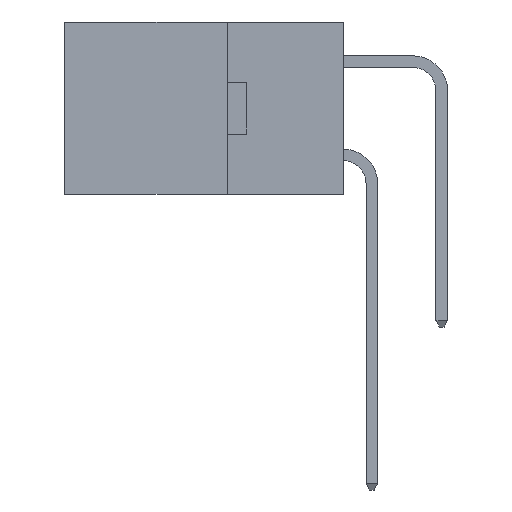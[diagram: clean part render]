
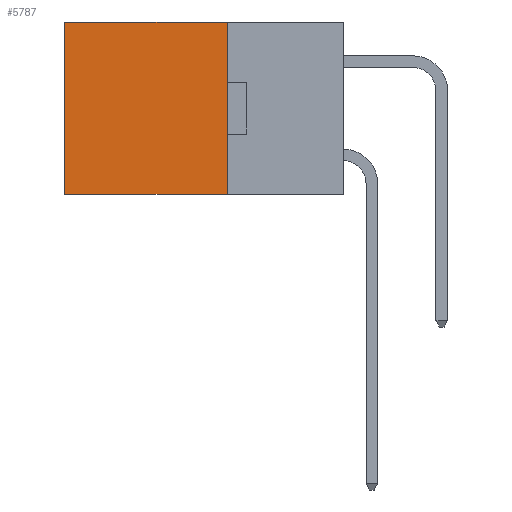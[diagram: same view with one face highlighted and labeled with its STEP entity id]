
A CAD part, left-side view. The second image highlights one B-rep face of the part: STEP entity #5787.
In plain terms, the highlighted planar face has unit normal (-1, 0, 0).
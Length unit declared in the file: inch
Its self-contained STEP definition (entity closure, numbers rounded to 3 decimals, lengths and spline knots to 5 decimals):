
#448 = VECTOR ( 'NONE', #6393, 39.37008 ) ;
#754 = CARTESIAN_POINT ( 'NONE',  ( 0.2615, 0.6, -0.37 ) ) ;
#781 = PLANE ( 'NONE',  #26436 ) ;
#1574 = DIRECTION ( 'NONE',  ( 0., 0., -1. ) ) ;
#1735 = VECTOR ( 'NONE', #27092, 39.37008 ) ;
#2966 = DIRECTION ( 'NONE',  ( 0., 0., -1. ) ) ;
#4983 = EDGE_CURVE ( 'NONE', #16024, #9648, #23648, .T. ) ;
#5787 = ADVANCED_FACE ( 'NONE', ( #12707 ), #781, .F. ) ;
#6393 = DIRECTION ( 'NONE',  ( 0., 1., 0. ) ) ;
#7378 = CARTESIAN_POINT ( 'NONE',  ( 0.2615, 0.25, 0. ) ) ;
#8198 = CARTESIAN_POINT ( 'NONE',  ( 0.2615, 0.6, -0.37 ) ) ;
#8821 = EDGE_CURVE ( 'NONE', #16024, #17655, #15399, .T. ) ;
#8940 = EDGE_CURVE ( 'NONE', #17655, #9509, #13372, .T. ) ;
#8962 = ORIENTED_EDGE ( 'NONE', *, *, #23899, .T. ) ;
#9121 = ORIENTED_EDGE ( 'NONE', *, *, #8940, .F. ) ;
#9509 = VERTEX_POINT ( 'NONE', #754 ) ;
#9621 = VECTOR ( 'NONE', #20264, 39.37008 ) ;
#9648 = VERTEX_POINT ( 'NONE', #10023 ) ;
#10023 = CARTESIAN_POINT ( 'NONE',  ( 0.2615, 0.6, 0. ) ) ;
#12707 = FACE_OUTER_BOUND ( 'NONE', #27432, .T. ) ;
#13372 = LINE ( 'NONE', #16251, #1735 ) ;
#13696 = CARTESIAN_POINT ( 'NONE',  ( 0.2615, 0.25, -0.37 ) ) ;
#15399 = LINE ( 'NONE', #13696, #9621 ) ;
#16024 = VERTEX_POINT ( 'NONE', #7378 ) ;
#16054 = DIRECTION ( 'NONE',  ( 1., 0., 0. ) ) ;
#16251 = CARTESIAN_POINT ( 'NONE',  ( 0.2615, 0.25, -0.37 ) ) ;
#17254 = CARTESIAN_POINT ( 'NONE',  ( 0.2615, 0.25, 0. ) ) ;
#17543 = ORIENTED_EDGE ( 'NONE', *, *, #4983, .T. ) ;
#17655 = VERTEX_POINT ( 'NONE', #22309 ) ;
#19858 = LINE ( 'NONE', #8198, #25618 ) ;
#20264 = DIRECTION ( 'NONE',  ( 0., 0., -1. ) ) ;
#22309 = CARTESIAN_POINT ( 'NONE',  ( 0.2615, 0.25, -0.37 ) ) ;
#23648 = LINE ( 'NONE', #17254, #448 ) ;
#23899 = EDGE_CURVE ( 'NONE', #9648, #9509, #19858, .T. ) ;
#25618 = VECTOR ( 'NONE', #1574, 39.37008 ) ;
#26436 = AXIS2_PLACEMENT_3D ( 'NONE', #26889, #16054, #2966 ) ;
#26889 = CARTESIAN_POINT ( 'NONE',  ( 0.2615, 0.25, -0.37 ) ) ;
#27092 = DIRECTION ( 'NONE',  ( 0., 1., 0. ) ) ;
#27425 = ORIENTED_EDGE ( 'NONE', *, *, #8821, .F. ) ;
#27432 = EDGE_LOOP ( 'NONE', ( #8962, #9121, #27425, #17543 ) ) ;
